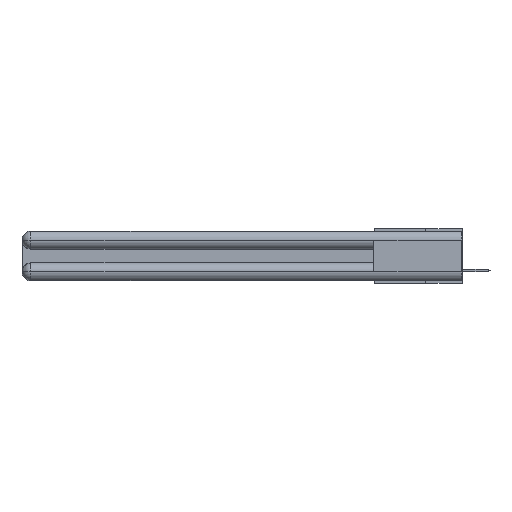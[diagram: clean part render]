
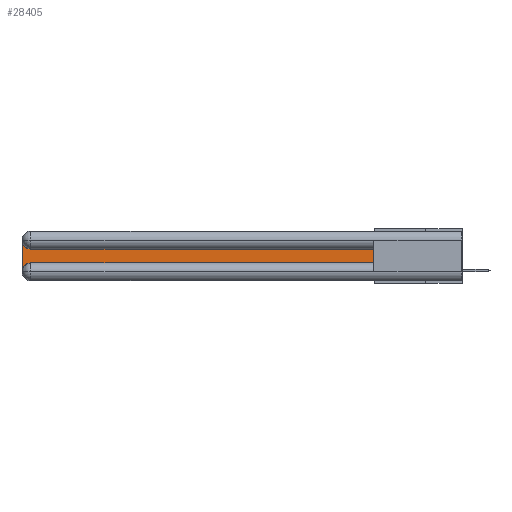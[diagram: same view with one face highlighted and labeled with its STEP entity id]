
A CAD part, left-side view. The second image highlights one B-rep face of the part: STEP entity #28405.
In plain terms, the highlighted planar face has unit normal (-1, 0, 0).
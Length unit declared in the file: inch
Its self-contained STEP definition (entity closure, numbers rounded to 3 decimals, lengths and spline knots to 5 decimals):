
#411 = CARTESIAN_POINT ( 'NONE',  ( 0.075, 2.94, -0.2775 ) ) ;
#449 = CARTESIAN_POINT ( 'NONE',  ( 0.075, 3., -0.1225 ) ) ;
#725 = LINE ( 'NONE', #12761, #25048 ) ;
#1188 = LINE ( 'NONE', #23785, #18645 ) ;
#1527 = EDGE_CURVE ( 'NONE', #12087, #5986, #725, .T. ) ;
#2184 = VERTEX_POINT ( 'NONE', #21872 ) ;
#2372 = EDGE_LOOP ( 'NONE', ( #14039, #20527, #26693, #6527, #11543, #12915 ) ) ;
#3161 = VECTOR ( 'NONE', #3384, 39.37008 ) ;
#3384 = DIRECTION ( 'NONE',  ( 0., -1., 0. ) ) ;
#4159 = DIRECTION ( 'NONE',  ( 0., 0., -1. ) ) ;
#4298 = CARTESIAN_POINT ( 'NONE',  ( 0.075, 0.6, -0.1225 ) ) ;
#4365 = AXIS2_PLACEMENT_3D ( 'NONE', #8480, #27505, #22887 ) ;
#4657 = CARTESIAN_POINT ( 'NONE',  ( 0.075, 3., -0.2775 ) ) ;
#5541 = EDGE_CURVE ( 'NONE', #2184, #10307, #21352, .T. ) ;
#5986 = VERTEX_POINT ( 'NONE', #4657 ) ;
#6527 = ORIENTED_EDGE ( 'NONE', *, *, #9402, .T. ) ;
#6893 = CARTESIAN_POINT ( 'NONE',  ( 0.075, 0.6, -0.2175 ) ) ;
#8219 = PLANE ( 'NONE',  #16920 ) ;
#8480 = CARTESIAN_POINT ( 'NONE',  ( 0.075, 2.94, -0.0625 ) ) ;
#8943 = DIRECTION ( 'NONE',  ( 1., 0., 0. ) ) ;
#9402 = EDGE_CURVE ( 'NONE', #5986, #2184, #11027, .T. ) ;
#9536 = VECTOR ( 'NONE', #28669, 39.37008 ) ;
#10307 = VERTEX_POINT ( 'NONE', #6893 ) ;
#10484 = EDGE_CURVE ( 'NONE', #13260, #12087, #19456, .T. ) ;
#10918 = EDGE_CURVE ( 'NONE', #10307, #18410, #1188, .T. ) ;
#11027 = CIRCLE ( 'NONE', #26941, 0.06 ) ;
#11298 = EDGE_CURVE ( 'NONE', #18410, #13260, #12925, .T. ) ;
#11543 = ORIENTED_EDGE ( 'NONE', *, *, #5541, .T. ) ;
#12087 = VERTEX_POINT ( 'NONE', #22301 ) ;
#12761 = CARTESIAN_POINT ( 'NONE',  ( 0.075, 3., -0.2175 ) ) ;
#12915 = ORIENTED_EDGE ( 'NONE', *, *, #10918, .T. ) ;
#12925 = LINE ( 'NONE', #13857, #9536 ) ;
#13260 = VERTEX_POINT ( 'NONE', #19595 ) ;
#13857 = CARTESIAN_POINT ( 'NONE',  ( 0.075, 0.6, -0.1225 ) ) ;
#14039 = ORIENTED_EDGE ( 'NONE', *, *, #11298, .T. ) ;
#16920 = AXIS2_PLACEMENT_3D ( 'NONE', #449, #8943, #4159 ) ;
#17965 = CARTESIAN_POINT ( 'NONE',  ( 0.075, 0.6, -0.2175 ) ) ;
#18410 = VERTEX_POINT ( 'NONE', #4298 ) ;
#18512 = FACE_OUTER_BOUND ( 'NONE', #2372, .T. ) ;
#18645 = VECTOR ( 'NONE', #21665, 39.37008 ) ;
#19456 = CIRCLE ( 'NONE', #4365, 0.06 ) ;
#19595 = CARTESIAN_POINT ( 'NONE',  ( 0.075, 2.94, -0.1225 ) ) ;
#20120 = DIRECTION ( 'NONE',  ( 0., 0., -1. ) ) ;
#20527 = ORIENTED_EDGE ( 'NONE', *, *, #10484, .T. ) ;
#21352 = LINE ( 'NONE', #17965, #3161 ) ;
#21665 = DIRECTION ( 'NONE',  ( 0., 0., 1. ) ) ;
#21872 = CARTESIAN_POINT ( 'NONE',  ( 0.075, 2.94, -0.2175 ) ) ;
#22301 = CARTESIAN_POINT ( 'NONE',  ( 0.075, 3., -0.0625 ) ) ;
#22687 = DIRECTION ( 'NONE',  ( 1., 0., 0. ) ) ;
#22887 = DIRECTION ( 'NONE',  ( 0., 0., -1. ) ) ;
#23785 = CARTESIAN_POINT ( 'NONE',  ( 0.075, 0.6, -0.2175 ) ) ;
#24728 = DIRECTION ( 'NONE',  ( 0., 0., -1. ) ) ;
#25048 = VECTOR ( 'NONE', #20120, 39.37008 ) ;
#26693 = ORIENTED_EDGE ( 'NONE', *, *, #1527, .T. ) ;
#26941 = AXIS2_PLACEMENT_3D ( 'NONE', #411, #22687, #24728 ) ;
#27505 = DIRECTION ( 'NONE',  ( 1., 0., 0. ) ) ;
#28405 = ADVANCED_FACE ( 'NONE', ( #18512 ), #8219, .F. ) ;
#28669 = DIRECTION ( 'NONE',  ( 0., 1., 0. ) ) ;
